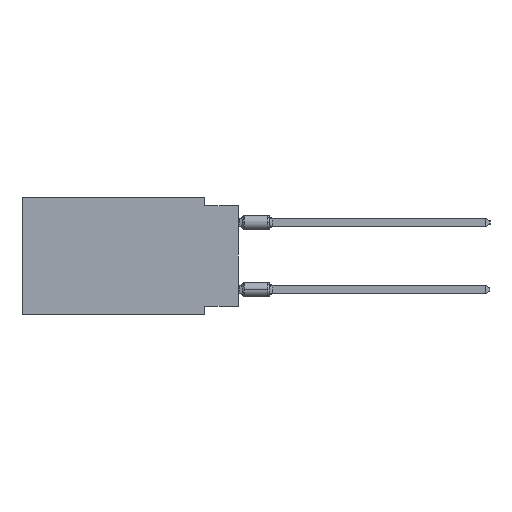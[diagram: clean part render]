
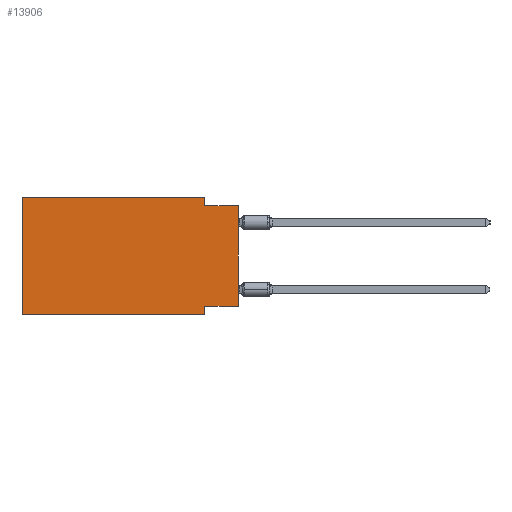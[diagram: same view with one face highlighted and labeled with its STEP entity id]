
A CAD part, left-side view. The second image highlights one B-rep face of the part: STEP entity #13906.
In plain terms, the highlighted planar face has unit normal (-1, 0, 0).
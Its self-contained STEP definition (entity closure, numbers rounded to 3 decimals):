
#1281 = VERTEX_POINT ( 'NONE', #26934 ) ;
#1683 = CARTESIAN_POINT ( 'NONE',  ( 0., 2.54, -8.255 ) ) ;
#2860 = ORIENTED_EDGE ( 'NONE', *, *, #3552, .F. ) ;
#3090 = LINE ( 'NONE', #18469, #21259 ) ;
#3552 = EDGE_CURVE ( 'NONE', #49840, #11307, #4808, .T. ) ;
#4808 = LINE ( 'NONE', #39891, #35422 ) ;
#5238 = LINE ( 'NONE', #24182, #16410 ) ;
#5354 = DIRECTION ( 'NONE',  ( 0., 0., -1. ) ) ;
#6571 = DIRECTION ( 'NONE',  ( 0., -1., 0. ) ) ;
#8485 = DIRECTION ( 'NONE',  ( 0., 0., 1. ) ) ;
#9190 = DIRECTION ( 'NONE',  ( 1., 0., 0. ) ) ;
#11276 = DIRECTION ( 'NONE',  ( 0., 0., -1. ) ) ;
#11307 = VERTEX_POINT ( 'NONE', #1683 ) ;
#11403 = EDGE_LOOP ( 'NONE', ( #27595, #36094, #31354, #15998, #24834, #36308, #45498, #2860 ) ) ;
#12772 = AXIS2_PLACEMENT_3D ( 'NONE', #16864, #9190, #5354 ) ;
#13906 = ADVANCED_FACE ( 'NONE', ( #24034 ), #36612, .F. ) ;
#14683 = VECTOR ( 'NONE', #6571, 1000. ) ;
#15002 = CARTESIAN_POINT ( 'NONE',  ( 0., 2.54, -8.89 ) ) ;
#15998 = ORIENTED_EDGE ( 'NONE', *, *, #31549, .F. ) ;
#16410 = VECTOR ( 'NONE', #44148, 1000. ) ;
#16864 = CARTESIAN_POINT ( 'NONE',  ( 0., 16.383, 0. ) ) ;
#18116 = DIRECTION ( 'NONE',  ( 0., -1., 0. ) ) ;
#18469 = CARTESIAN_POINT ( 'NONE',  ( 0., 2.54, -8.89 ) ) ;
#21259 = VECTOR ( 'NONE', #33347, 1000. ) ;
#22120 = CARTESIAN_POINT ( 'NONE',  ( 0., 2.54, -0.635 ) ) ;
#24034 = FACE_OUTER_BOUND ( 'NONE', #11403, .T. ) ;
#24182 = CARTESIAN_POINT ( 'NONE',  ( 0., 0., 0. ) ) ;
#24834 = ORIENTED_EDGE ( 'NONE', *, *, #41953, .F. ) ;
#25166 = VECTOR ( 'NONE', #18116, 1000. ) ;
#25274 = VECTOR ( 'NONE', #45005, 1000. ) ;
#25284 = DIRECTION ( 'NONE',  ( 0., 1., 0. ) ) ;
#25797 = CARTESIAN_POINT ( 'NONE',  ( 0., 0., -0.635 ) ) ;
#26934 = CARTESIAN_POINT ( 'NONE',  ( 0., 16.383, -8.89 ) ) ;
#27595 = ORIENTED_EDGE ( 'NONE', *, *, #45616, .T. ) ;
#28720 = LINE ( 'NONE', #36155, #31347 ) ;
#29407 = LINE ( 'NONE', #29654, #25274 ) ;
#29654 = CARTESIAN_POINT ( 'NONE',  ( 0., 16.383, 0. ) ) ;
#30244 = EDGE_CURVE ( 'NONE', #42977, #39489, #33757, .T. ) ;
#30639 = CARTESIAN_POINT ( 'NONE',  ( 0., 2.54, 0. ) ) ;
#31347 = VECTOR ( 'NONE', #8485, 1000. ) ;
#31354 = ORIENTED_EDGE ( 'NONE', *, *, #43444, .F. ) ;
#31496 = VERTEX_POINT ( 'NONE', #48848 ) ;
#31549 = EDGE_CURVE ( 'NONE', #31496, #39651, #29407, .T. ) ;
#33347 = DIRECTION ( 'NONE',  ( 0., 0., -1. ) ) ;
#33757 = LINE ( 'NONE', #25797, #25166 ) ;
#35422 = VECTOR ( 'NONE', #25284, 1000. ) ;
#36094 = ORIENTED_EDGE ( 'NONE', *, *, #30244, .F. ) ;
#36109 = CARTESIAN_POINT ( 'NONE',  ( 0., 0., -8.255 ) ) ;
#36155 = CARTESIAN_POINT ( 'NONE',  ( 0., 16.383, 0. ) ) ;
#36308 = ORIENTED_EDGE ( 'NONE', *, *, #42498, .T. ) ;
#36612 = PLANE ( 'NONE',  #12772 ) ;
#39297 = VECTOR ( 'NONE', #11276, 1000. ) ;
#39489 = VERTEX_POINT ( 'NONE', #49065 ) ;
#39591 = VERTEX_POINT ( 'NONE', #15002 ) ;
#39651 = VERTEX_POINT ( 'NONE', #30639 ) ;
#39891 = CARTESIAN_POINT ( 'NONE',  ( 0., 0., -8.255 ) ) ;
#41953 = EDGE_CURVE ( 'NONE', #1281, #31496, #28720, .T. ) ;
#42498 = EDGE_CURVE ( 'NONE', #1281, #39591, #45980, .T. ) ;
#42514 = CARTESIAN_POINT ( 'NONE',  ( 0., 2.54, 0. ) ) ;
#42977 = VERTEX_POINT ( 'NONE', #22120 ) ;
#43250 = EDGE_CURVE ( 'NONE', #11307, #39591, #3090, .T. ) ;
#43444 = EDGE_CURVE ( 'NONE', #39651, #42977, #47339, .T. ) ;
#44148 = DIRECTION ( 'NONE',  ( 0., 0., 1. ) ) ;
#45005 = DIRECTION ( 'NONE',  ( 0., -1., 0. ) ) ;
#45498 = ORIENTED_EDGE ( 'NONE', *, *, #43250, .F. ) ;
#45616 = EDGE_CURVE ( 'NONE', #49840, #39489, #5238, .T. ) ;
#45980 = LINE ( 'NONE', #50310, #14683 ) ;
#47339 = LINE ( 'NONE', #42514, #39297 ) ;
#48848 = CARTESIAN_POINT ( 'NONE',  ( 0., 16.383, 0. ) ) ;
#49065 = CARTESIAN_POINT ( 'NONE',  ( 0., 0., -0.635 ) ) ;
#49840 = VERTEX_POINT ( 'NONE', #36109 ) ;
#50310 = CARTESIAN_POINT ( 'NONE',  ( 0., 16.383, -8.89 ) ) ;
